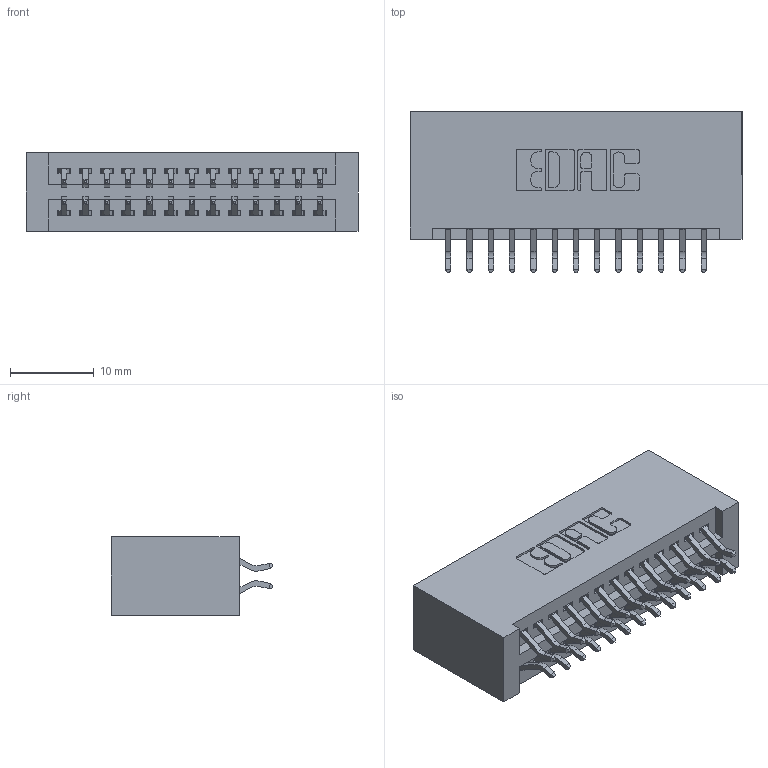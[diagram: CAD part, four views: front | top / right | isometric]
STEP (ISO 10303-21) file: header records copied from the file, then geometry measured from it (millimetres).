
FILE_DESCRIPTION (( 'STEP AP203' ), '1' );
FILE_NAME ('345-026-556-201.STEP', '2018-08-22T03:09:53', ( '' ), ( '' ), 'SwSTEP 2.0', 'SolidWorks 2016', '' );
FILE_SCHEMA (( 'CONFIG_CONTROL_DESIGN' ));
Length unit declared in the file: inch
Products named in the file (3): 345 Part_No Mounting Lugs; 345-292-001_556 Tail; 345-026-556-201
Assembly tree (27 placements, depth 2):
  345-026-556-201
    345 Part_No Mounting Lugs
    345-292-001_556 Tail  x26
Bounding box: 39.62 x 19.24 x 9.4 mm (x, y, z)
Volume: 4194.8 mm3; surface area: 5919.5 mm2
Topology: 27 solids, 27 shells, 1574 faces, 4659 edges, 3070 vertices
Faces by surface type: plane 1038, cylinder 536
Entity records: 14047 total; most frequent: CARTESIAN_POINT 2396, ORIENTED_EDGE 2318, DIRECTION 2131, EDGE_CURVE 1159, LINE 975, VECTOR 975, VERTEX_POINT 770, AXIS2_PLACEMENT_3D 578
